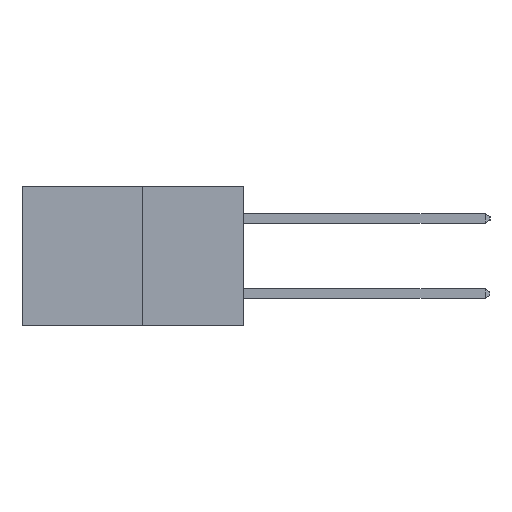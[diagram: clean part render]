
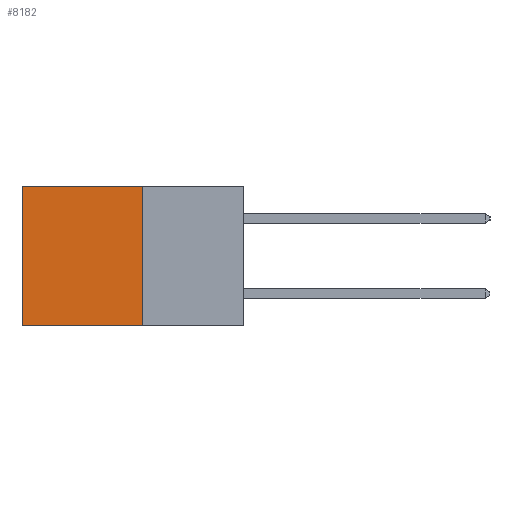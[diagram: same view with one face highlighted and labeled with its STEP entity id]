
A CAD part, left-side view. The second image highlights one B-rep face of the part: STEP entity #8182.
In plain terms, the highlighted planar face has unit normal (-1, 0, 0).
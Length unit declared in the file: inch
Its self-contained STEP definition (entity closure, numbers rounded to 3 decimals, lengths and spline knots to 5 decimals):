
#900 = CARTESIAN_POINT ( 'NONE',  ( 0.277, 0.27, -0.37 ) ) ;
#2910 = CARTESIAN_POINT ( 'NONE',  ( 0.277, 0.59, 0. ) ) ;
#3084 = ORIENTED_EDGE ( 'NONE', *, *, #21791, .T. ) ;
#3637 = CARTESIAN_POINT ( 'NONE',  ( 0.277, 0.27, -0.37 ) ) ;
#3720 = DIRECTION ( 'NONE',  ( 1., 0., 0. ) ) ;
#3841 = DIRECTION ( 'NONE',  ( 0., 0., -1. ) ) ;
#3982 = CARTESIAN_POINT ( 'NONE',  ( 0.277, 0.27, -0.37 ) ) ;
#4152 = PLANE ( 'NONE',  #7002 ) ;
#7002 = AXIS2_PLACEMENT_3D ( 'NONE', #3982, #3720, #3841 ) ;
#8182 = ADVANCED_FACE ( 'NONE', ( #16579 ), #4152, .F. ) ;
#8822 = CARTESIAN_POINT ( 'NONE',  ( 0.277, 0.27, 0. ) ) ;
#9347 = LINE ( 'NONE', #900, #22197 ) ;
#10354 = VERTEX_POINT ( 'NONE', #2910 ) ;
#11541 = VECTOR ( 'NONE', #21122, 39.37008 ) ;
#11973 = EDGE_LOOP ( 'NONE', ( #22386, #15987, #14038, #3084 ) ) ;
#12588 = DIRECTION ( 'NONE',  ( 0., 0., -1. ) ) ;
#14038 = ORIENTED_EDGE ( 'NONE', *, *, #19536, .F. ) ;
#14405 = CARTESIAN_POINT ( 'NONE',  ( 0.277, 0.59, -0.37 ) ) ;
#15038 = CARTESIAN_POINT ( 'NONE',  ( 0.277, 0.27, -0.37 ) ) ;
#15987 = ORIENTED_EDGE ( 'NONE', *, *, #20211, .F. ) ;
#16579 = FACE_OUTER_BOUND ( 'NONE', #11973, .T. ) ;
#16704 = LINE ( 'NONE', #14405, #20205 ) ;
#16859 = DIRECTION ( 'NONE',  ( 0., 1., 0. ) ) ;
#17426 = LINE ( 'NONE', #15038, #21391 ) ;
#17852 = VERTEX_POINT ( 'NONE', #3637 ) ;
#17888 = EDGE_CURVE ( 'NONE', #10354, #19189, #16704, .T. ) ;
#19189 = VERTEX_POINT ( 'NONE', #21203 ) ;
#19536 = EDGE_CURVE ( 'NONE', #22066, #17852, #9347, .T. ) ;
#20094 = CARTESIAN_POINT ( 'NONE',  ( 0.277, 0.27, 0. ) ) ;
#20205 = VECTOR ( 'NONE', #12588, 39.37008 ) ;
#20211 = EDGE_CURVE ( 'NONE', #17852, #19189, #17426, .T. ) ;
#20313 = LINE ( 'NONE', #8822, #11541 ) ;
#20465 = DIRECTION ( 'NONE',  ( 0., 0., -1. ) ) ;
#21122 = DIRECTION ( 'NONE',  ( 0., 1., 0. ) ) ;
#21203 = CARTESIAN_POINT ( 'NONE',  ( 0.277, 0.59, -0.37 ) ) ;
#21391 = VECTOR ( 'NONE', #16859, 39.37008 ) ;
#21791 = EDGE_CURVE ( 'NONE', #22066, #10354, #20313, .T. ) ;
#22066 = VERTEX_POINT ( 'NONE', #20094 ) ;
#22197 = VECTOR ( 'NONE', #20465, 39.37008 ) ;
#22386 = ORIENTED_EDGE ( 'NONE', *, *, #17888, .T. ) ;
